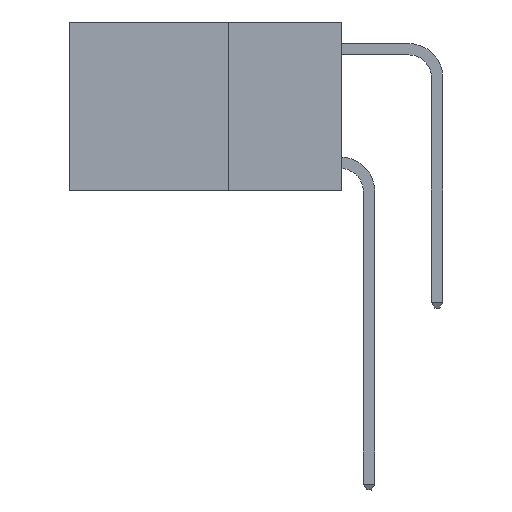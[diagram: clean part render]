
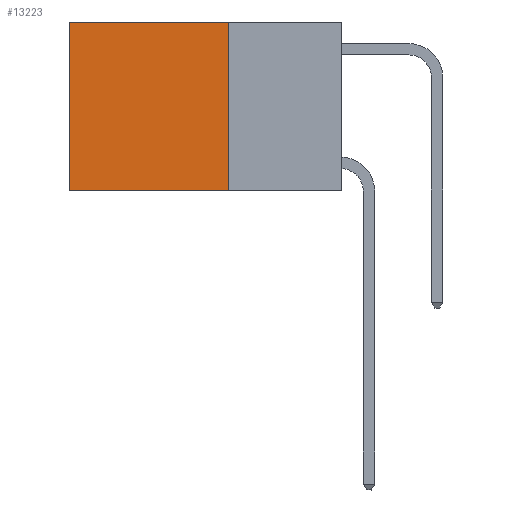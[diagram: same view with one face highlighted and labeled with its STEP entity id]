
A CAD part, left-side view. The second image highlights one B-rep face of the part: STEP entity #13223.
In plain terms, the highlighted planar face has unit normal (-1, 0, 0).
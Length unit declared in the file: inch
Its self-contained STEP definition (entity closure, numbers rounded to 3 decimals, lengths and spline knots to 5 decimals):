
#337 = ORIENTED_EDGE ( 'NONE', *, *, #7748, .T. ) ;
#550 = VECTOR ( 'NONE', #16416, 39.37008 ) ;
#1782 = LINE ( 'NONE', #15420, #7544 ) ;
#2767 = VECTOR ( 'NONE', #10014, 39.37008 ) ;
#2925 = DIRECTION ( 'NONE',  ( 0., 0., -1. ) ) ;
#4185 = ORIENTED_EDGE ( 'NONE', *, *, #13194, .F. ) ;
#4438 = CARTESIAN_POINT ( 'NONE',  ( 0.2625, 0.25, 0. ) ) ;
#4728 = FACE_OUTER_BOUND ( 'NONE', #11205, .T. ) ;
#5187 = ORIENTED_EDGE ( 'NONE', *, *, #18968, .T. ) ;
#6065 = CARTESIAN_POINT ( 'NONE',  ( 0.2625, 0.6, 0. ) ) ;
#6232 = PLANE ( 'NONE',  #21103 ) ;
#6497 = CARTESIAN_POINT ( 'NONE',  ( 0.2625, 0.25, 0. ) ) ;
#6977 = LINE ( 'NONE', #6497, #2767 ) ;
#7544 = VECTOR ( 'NONE', #10217, 39.37008 ) ;
#7748 = EDGE_CURVE ( 'NONE', #16421, #20628, #1782, .T. ) ;
#8744 = EDGE_CURVE ( 'NONE', #12169, #21242, #6977, .T. ) ;
#9651 = CARTESIAN_POINT ( 'NONE',  ( 0.2625, 0.25, 0. ) ) ;
#10014 = DIRECTION ( 'NONE',  ( 0., 0., -1. ) ) ;
#10217 = DIRECTION ( 'NONE',  ( 0., 0., -1. ) ) ;
#10366 = CARTESIAN_POINT ( 'NONE',  ( 0.2625, 0.25, -0.37 ) ) ;
#10747 = LINE ( 'NONE', #4438, #20861 ) ;
#11205 = EDGE_LOOP ( 'NONE', ( #337, #4185, #20647, #5187 ) ) ;
#12169 = VERTEX_POINT ( 'NONE', #9651 ) ;
#12984 = DIRECTION ( 'NONE',  ( 1., 0., 0. ) ) ;
#13194 = EDGE_CURVE ( 'NONE', #21242, #20628, #14164, .T. ) ;
#13223 = ADVANCED_FACE ( 'NONE', ( #4728 ), #6232, .F. ) ;
#14164 = LINE ( 'NONE', #19428, #550 ) ;
#15420 = CARTESIAN_POINT ( 'NONE',  ( 0.2625, 0.6, 0. ) ) ;
#16416 = DIRECTION ( 'NONE',  ( 0., 1., 0. ) ) ;
#16421 = VERTEX_POINT ( 'NONE', #6065 ) ;
#18026 = CARTESIAN_POINT ( 'NONE',  ( 0.2625, 0.25, 0. ) ) ;
#18968 = EDGE_CURVE ( 'NONE', #12169, #16421, #10747, .T. ) ;
#19336 = DIRECTION ( 'NONE',  ( 0., 1., 0. ) ) ;
#19428 = CARTESIAN_POINT ( 'NONE',  ( 0.2625, 0.25, -0.37 ) ) ;
#20628 = VERTEX_POINT ( 'NONE', #20736 ) ;
#20647 = ORIENTED_EDGE ( 'NONE', *, *, #8744, .F. ) ;
#20736 = CARTESIAN_POINT ( 'NONE',  ( 0.2625, 0.6, -0.37 ) ) ;
#20861 = VECTOR ( 'NONE', #19336, 39.37008 ) ;
#21103 = AXIS2_PLACEMENT_3D ( 'NONE', #18026, #12984, #2925 ) ;
#21242 = VERTEX_POINT ( 'NONE', #10366 ) ;
